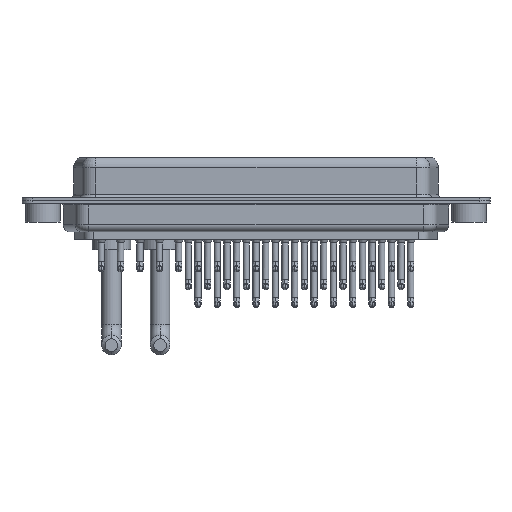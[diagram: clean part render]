
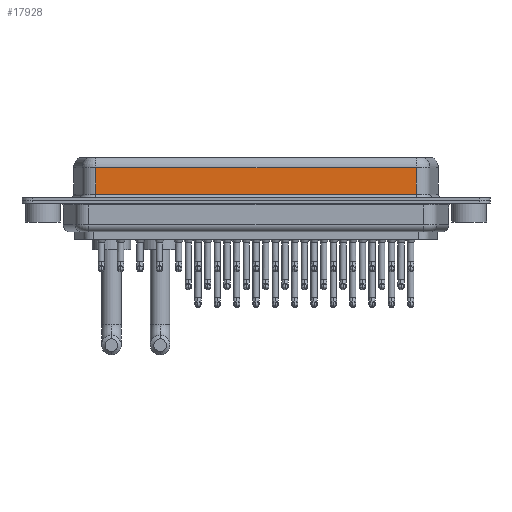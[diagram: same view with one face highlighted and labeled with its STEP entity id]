
A CAD part, front view. The second image highlights one B-rep face of the part: STEP entity #17928.
In plain terms, the highlighted planar face has unit normal (0, -1, 0).
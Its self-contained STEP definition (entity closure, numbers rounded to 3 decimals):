
#600 = ORIENTED_EDGE ( 'NONE', *, *, #1077, .F. ) ;
#1077 = EDGE_CURVE ( 'NONE', #27374, #9460, #21902, .T. ) ;
#2061 = DIRECTION ( 'NONE',  ( 1., 0., 0. ) ) ;
#2358 = DIRECTION ( 'NONE',  ( 0., 0., -1. ) ) ;
#2374 = ORIENTED_EDGE ( 'NONE', *, *, #30388, .T. ) ;
#2550 = CARTESIAN_POINT ( 'NONE',  ( 53.41, -5.375, 0.9 ) ) ;
#4623 = ORIENTED_EDGE ( 'NONE', *, *, #14092, .T. ) ;
#4770 = LINE ( 'NONE', #6593, #19923 ) ;
#6164 = EDGE_LOOP ( 'NONE', ( #600, #6453, #2374, #4623 ) ) ;
#6398 = VERTEX_POINT ( 'NONE', #7321 ) ;
#6453 = ORIENTED_EDGE ( 'NONE', *, *, #26940, .T. ) ;
#6593 = CARTESIAN_POINT ( 'NONE',  ( 7.59, -5.375, 6.4 ) ) ;
#7151 = LINE ( 'NONE', #2550, #23933 ) ;
#7321 = CARTESIAN_POINT ( 'NONE',  ( 7.59, -5.375, 4.65 ) ) ;
#8224 = DIRECTION ( 'NONE',  ( 0., 1., 0. ) ) ;
#8592 = CARTESIAN_POINT ( 'NONE',  ( 7.59, -5.375, 0.9 ) ) ;
#9460 = VERTEX_POINT ( 'NONE', #20947 ) ;
#10690 = FACE_OUTER_BOUND ( 'NONE', #6164, .T. ) ;
#10930 = DIRECTION ( 'NONE',  ( -1., 0., 0. ) ) ;
#14092 = EDGE_CURVE ( 'NONE', #19755, #9460, #7151, .T. ) ;
#15776 = DIRECTION ( 'NONE',  ( 0., 0., 1. ) ) ;
#16607 = DIRECTION ( 'NONE',  ( 0., 0., -1. ) ) ;
#17276 = VECTOR ( 'NONE', #2358, 1000. ) ;
#17928 = ADVANCED_FACE ( 'NONE', ( #10690 ), #31062, .F. ) ;
#17988 = CARTESIAN_POINT ( 'NONE',  ( 53.41, -5.375, 4.65 ) ) ;
#18479 = LINE ( 'NONE', #17988, #31362 ) ;
#19755 = VERTEX_POINT ( 'NONE', #8592 ) ;
#19923 = VECTOR ( 'NONE', #16607, 1000. ) ;
#20947 = CARTESIAN_POINT ( 'NONE',  ( 53.41, -5.375, 0.9 ) ) ;
#21902 = LINE ( 'NONE', #29637, #17276 ) ;
#23933 = VECTOR ( 'NONE', #2061, 1000. ) ;
#26280 = AXIS2_PLACEMENT_3D ( 'NONE', #30740, #8224, #15776 ) ;
#26940 = EDGE_CURVE ( 'NONE', #27374, #6398, #18479, .T. ) ;
#27374 = VERTEX_POINT ( 'NONE', #30100 ) ;
#29637 = CARTESIAN_POINT ( 'NONE',  ( 53.41, -5.375, 6.4 ) ) ;
#30100 = CARTESIAN_POINT ( 'NONE',  ( 53.41, -5.375, 4.65 ) ) ;
#30388 = EDGE_CURVE ( 'NONE', #6398, #19755, #4770, .T. ) ;
#30740 = CARTESIAN_POINT ( 'NONE',  ( 53.41, -5.375, 6.4 ) ) ;
#31062 = PLANE ( 'NONE',  #26280 ) ;
#31362 = VECTOR ( 'NONE', #10930, 1000. ) ;
